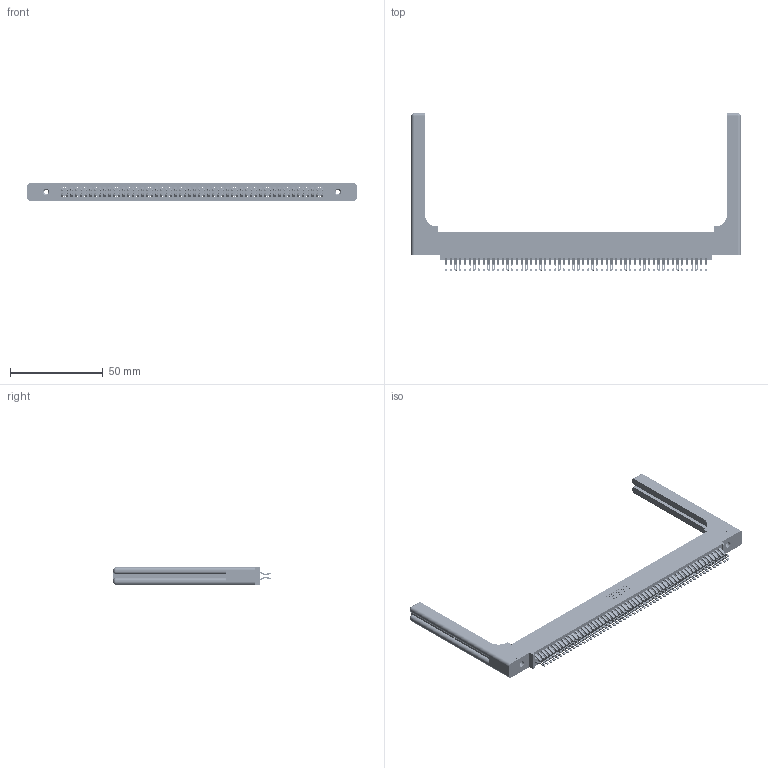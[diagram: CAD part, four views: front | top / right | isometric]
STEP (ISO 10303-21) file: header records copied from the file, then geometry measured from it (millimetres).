
FILE_DESCRIPTION (( 'STEP AP203' ), '1' );
FILE_NAME ('395-112-555-558.STEP', '2019-10-27T15:56:34', ( '' ), ( '' ), 'SwSTEP 2.0', 'SolidWorks 2016', '' );
FILE_SCHEMA (( 'CONFIG_CONTROL_DESIGN' ));
Length unit declared in the file: inch
Products named in the file (5): 345-220-058_345-220-058; 395-112-555-558; 345 Part_0.110 Offset - 0.156 Dia-TH; 345-292-001_555 Tail; 345-250-001_345-250-001-102
Assembly tree (117 placements, depth 2):
  395-112-555-558
    345 Part_0.110 Offset - 0.156 Dia-TH
    345-292-001_555 Tail  x112
    345-250-001_345-250-001-102  x2
    345-220-058_345-220-058  x2
Bounding box: 177.27 x 84.89 x 9.4 mm (x, y, z)
Volume: 26076.4 mm3; surface area: 32570.4 mm2
Topology: 117 solids, 117 shells, 6658 faces, 20843 edges, 13874 vertices
Faces by surface type: plane 3704, cylinder 2894, bspline 36, cone 12, sphere 8, torus 4
Entity records: 47694 total; most frequent: CARTESIAN_POINT 9011, ORIENTED_EDGE 7712, DIRECTION 6828, EDGE_CURVE 3856, LINE 3388, VECTOR 3388, VERTEX_POINT 2562, AXIS2_PLACEMENT_3D 1720
